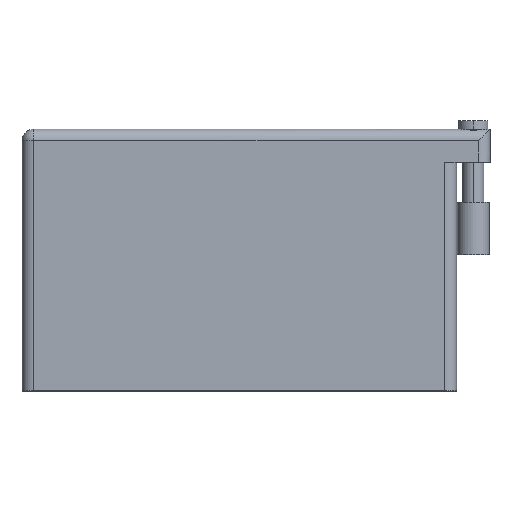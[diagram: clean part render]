
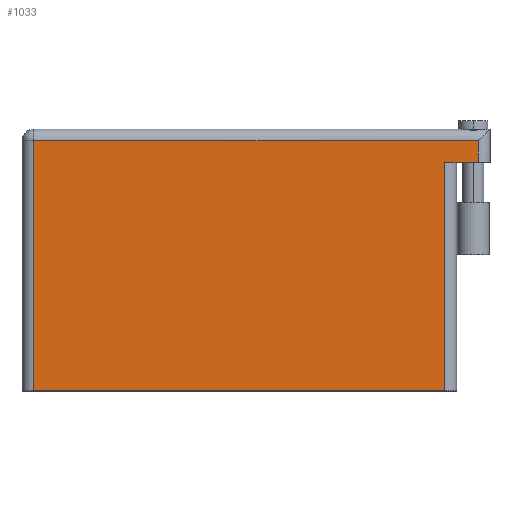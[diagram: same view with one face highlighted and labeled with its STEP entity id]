
A CAD part, top view. The second image highlights one B-rep face of the part: STEP entity #1033.
In plain terms, the highlighted planar face has unit normal (0, 0, 1).
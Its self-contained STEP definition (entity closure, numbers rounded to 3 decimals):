
#15 = CARTESIAN_POINT ( 'NONE',  ( 69.342, 37.998, 0. ) ) ;
#48 = CARTESIAN_POINT ( 'NONE',  ( 1.778, 0., 0. ) ) ;
#69 = EDGE_CURVE ( 'NONE', #1903, #1114, #217, .T. ) ;
#127 = VERTEX_POINT ( 'NONE', #1293 ) ;
#217 = LINE ( 'NONE', #48, #659 ) ;
#239 = CARTESIAN_POINT ( 'NONE',  ( 69.342, 34.773, 0. ) ) ;
#279 = VERTEX_POINT ( 'NONE', #1591 ) ;
#401 = LINE ( 'NONE', #1126, #1558 ) ;
#449 = CARTESIAN_POINT ( 'NONE',  ( 1.778, 37.998, 0. ) ) ;
#472 = ORIENTED_EDGE ( 'NONE', *, *, #830, .T. ) ;
#484 = DIRECTION ( 'NONE',  ( -1., 0., 0. ) ) ;
#491 = LINE ( 'NONE', #984, #1739 ) ;
#659 = VECTOR ( 'NONE', #720, 1000. ) ;
#720 = DIRECTION ( 'NONE',  ( 0., -1., 0. ) ) ;
#738 = ORIENTED_EDGE ( 'NONE', *, *, #1290, .T. ) ;
#782 = EDGE_CURVE ( 'NONE', #1154, #127, #1121, .T. ) ;
#786 = CARTESIAN_POINT ( 'NONE',  ( 1.778, 0., 0. ) ) ;
#794 = DIRECTION ( 'NONE',  ( 0., 1., 0. ) ) ;
#830 = EDGE_CURVE ( 'NONE', #1154, #2044, #1953, .T. ) ;
#880 = VECTOR ( 'NONE', #484, 1000. ) ;
#967 = CARTESIAN_POINT ( 'NONE',  ( 71.12, 34.773, 0. ) ) ;
#984 = CARTESIAN_POINT ( 'NONE',  ( 64.262, 34.773, 0. ) ) ;
#1033 = ADVANCED_FACE ( 'NONE', ( #1209 ), #1552, .F. ) ;
#1114 = VERTEX_POINT ( 'NONE', #786 ) ;
#1121 = LINE ( 'NONE', #967, #1445 ) ;
#1126 = CARTESIAN_POINT ( 'NONE',  ( 0., 0., 0. ) ) ;
#1152 = EDGE_LOOP ( 'NONE', ( #738, #1706, #2075, #472, #1782, #1623 ) ) ;
#1154 = VERTEX_POINT ( 'NONE', #239 ) ;
#1156 = AXIS2_PLACEMENT_3D ( 'NONE', #1726, #1220, #1910 ) ;
#1209 = FACE_OUTER_BOUND ( 'NONE', #1152, .T. ) ;
#1220 = DIRECTION ( 'NONE',  ( 0., 0., -1. ) ) ;
#1290 = EDGE_CURVE ( 'NONE', #1114, #279, #401, .T. ) ;
#1293 = CARTESIAN_POINT ( 'NONE',  ( 64.262, 34.773, 0. ) ) ;
#1298 = CARTESIAN_POINT ( 'NONE',  ( 69.342, 39.776, 0. ) ) ;
#1329 = VECTOR ( 'NONE', #1447, 1000. ) ;
#1367 = LINE ( 'NONE', #2179, #880 ) ;
#1386 = EDGE_CURVE ( 'NONE', #2044, #1903, #1367, .T. ) ;
#1445 = VECTOR ( 'NONE', #2115, 1000. ) ;
#1447 = DIRECTION ( 'NONE',  ( 0., 1., 0. ) ) ;
#1552 = PLANE ( 'NONE',  #1156 ) ;
#1558 = VECTOR ( 'NONE', #1990, 1000. ) ;
#1591 = CARTESIAN_POINT ( 'NONE',  ( 64.262, 0., 0. ) ) ;
#1623 = ORIENTED_EDGE ( 'NONE', *, *, #69, .T. ) ;
#1689 = EDGE_CURVE ( 'NONE', #279, #127, #491, .T. ) ;
#1706 = ORIENTED_EDGE ( 'NONE', *, *, #1689, .T. ) ;
#1726 = CARTESIAN_POINT ( 'NONE',  ( 0., 39.776, 0. ) ) ;
#1739 = VECTOR ( 'NONE', #794, 1000. ) ;
#1782 = ORIENTED_EDGE ( 'NONE', *, *, #1386, .T. ) ;
#1903 = VERTEX_POINT ( 'NONE', #449 ) ;
#1910 = DIRECTION ( 'NONE',  ( -1., 0., 0. ) ) ;
#1953 = LINE ( 'NONE', #1298, #1329 ) ;
#1990 = DIRECTION ( 'NONE',  ( 1., 0., 0. ) ) ;
#2044 = VERTEX_POINT ( 'NONE', #15 ) ;
#2075 = ORIENTED_EDGE ( 'NONE', *, *, #782, .F. ) ;
#2115 = DIRECTION ( 'NONE',  ( -1., 0., 0. ) ) ;
#2179 = CARTESIAN_POINT ( 'NONE',  ( 0., 37.998, 0. ) ) ;
